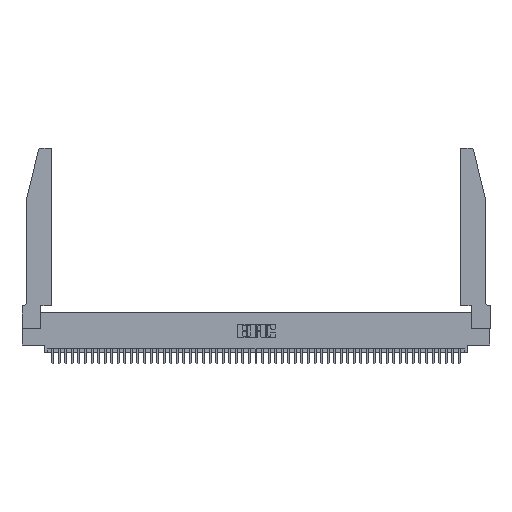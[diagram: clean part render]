
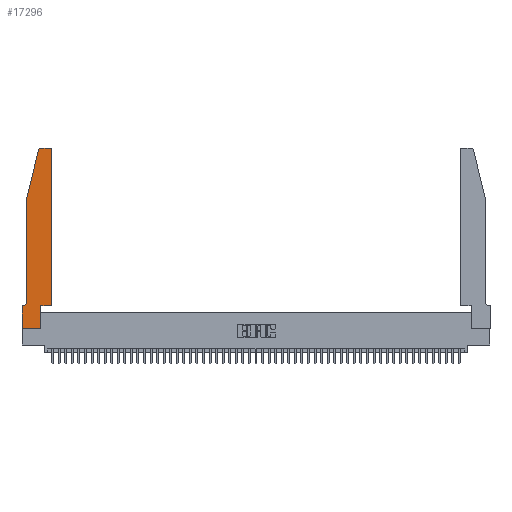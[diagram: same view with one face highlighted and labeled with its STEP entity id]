
A CAD part, top view. The second image highlights one B-rep face of the part: STEP entity #17296.
In plain terms, the highlighted planar face has unit normal (0, 0, 1).
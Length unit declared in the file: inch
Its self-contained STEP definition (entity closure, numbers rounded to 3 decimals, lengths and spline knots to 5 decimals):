
#713 = ORIENTED_EDGE ( 'NONE', *, *, #47006, .T. ) ;
#807 = EDGE_CURVE ( 'NONE', #51431, #30269, #21601, .T. ) ;
#2073 = ORIENTED_EDGE ( 'NONE', *, *, #3353, .T. ) ;
#3353 = EDGE_CURVE ( 'NONE', #23735, #6750, #13855, .T. ) ;
#3904 = VERTEX_POINT ( 'NONE', #6101 ) ;
#3996 = DIRECTION ( 'NONE',  ( 0., -1., 0. ) ) ;
#4215 = CARTESIAN_POINT ( 'NONE',  ( 0.0755, 2., 0.37 ) ) ;
#4515 = VERTEX_POINT ( 'NONE', #13367 ) ;
#4676 = CARTESIAN_POINT ( 'NONE',  ( 0.0755, 0.35, 0.37 ) ) ;
#4972 = CARTESIAN_POINT ( 'NONE',  ( 0.2865, 0.35, 0.37 ) ) ;
#5237 = PLANE ( 'NONE',  #23250 ) ;
#5437 = DIRECTION ( 'NONE',  ( 1., 0., 0. ) ) ;
#5572 = CARTESIAN_POINT ( 'NONE',  ( 0., 0., 0.37 ) ) ;
#5615 = DIRECTION ( 'NONE',  ( 0., 0., -1. ) ) ;
#5679 = DIRECTION ( 'NONE',  ( 1., 0., 0. ) ) ;
#5750 = ORIENTED_EDGE ( 'NONE', *, *, #49081, .T. ) ;
#6101 = CARTESIAN_POINT ( 'NONE',  ( 0.284, 2.75, 0.37 ) ) ;
#6127 = EDGE_CURVE ( 'NONE', #3904, #4515, #20749, .T. ) ;
#6750 = VERTEX_POINT ( 'NONE', #40614 ) ;
#6787 = CARTESIAN_POINT ( 'NONE',  ( 0.4505, 2.72, 0.37 ) ) ;
#8345 = EDGE_LOOP ( 'NONE', ( #8505, #27759, #46251, #5750, #2073, #32078, #30942, #51283, #11053, #10192, #48092, #713 ) ) ;
#8505 = ORIENTED_EDGE ( 'NONE', *, *, #30187, .T. ) ;
#8532 = CARTESIAN_POINT ( 'NONE',  ( 0.4205, 2.75, 0.37 ) ) ;
#9733 = EDGE_CURVE ( 'NONE', #40863, #49218, #51034, .T. ) ;
#9951 = CARTESIAN_POINT ( 'NONE',  ( 0.4205, 2.72, 0.37 ) ) ;
#10105 = LINE ( 'NONE', #41213, #39370 ) ;
#10192 = ORIENTED_EDGE ( 'NONE', *, *, #43537, .T. ) ;
#10645 = DIRECTION ( 'NONE',  ( 0., 0., 1. ) ) ;
#10842 = CARTESIAN_POINT ( 'NONE',  ( 0.4505, 0.35, 0.37 ) ) ;
#11053 = ORIENTED_EDGE ( 'NONE', *, *, #9733, .T. ) ;
#13268 = CARTESIAN_POINT ( 'NONE',  ( 0., 0.35, 0.37 ) ) ;
#13367 = CARTESIAN_POINT ( 'NONE',  ( 0.25487, 2.72718, 0.37 ) ) ;
#13855 = CIRCLE ( 'NONE', #32529, 0.07 ) ;
#14423 = EDGE_CURVE ( 'NONE', #4515, #18937, #43116, .T. ) ;
#14826 = DIRECTION ( 'NONE',  ( -1., 0., 0. ) ) ;
#16550 = DIRECTION ( 'NONE',  ( -1., 0., 0. ) ) ;
#16943 = VECTOR ( 'NONE', #47960, 39.37008 ) ;
#17296 = ADVANCED_FACE ( 'NONE', ( #25912 ), #5237, .T. ) ;
#17378 = AXIS2_PLACEMENT_3D ( 'NONE', #9951, #10645, #30489 ) ;
#18166 = VERTEX_POINT ( 'NONE', #31479 ) ;
#18937 = VERTEX_POINT ( 'NONE', #27567 ) ;
#20621 = CARTESIAN_POINT ( 'NONE',  ( 0.4505, 0.35, 0.37 ) ) ;
#20661 = DIRECTION ( 'NONE',  ( 0., 1., 0. ) ) ;
#20749 = CIRCLE ( 'NONE', #22957, 0.03 ) ;
#21378 = DIRECTION ( 'NONE',  ( 0., -1., 0. ) ) ;
#21601 = LINE ( 'NONE', #20621, #49634 ) ;
#22957 = AXIS2_PLACEMENT_3D ( 'NONE', #35944, #49182, #5437 ) ;
#23005 = VECTOR ( 'NONE', #20661, 39.37008 ) ;
#23250 = AXIS2_PLACEMENT_3D ( 'NONE', #13268, #41106, #33295 ) ;
#23680 = EDGE_CURVE ( 'NONE', #42241, #40863, #33078, .T. ) ;
#23735 = VERTEX_POINT ( 'NONE', #34259 ) ;
#25087 = DIRECTION ( 'NONE',  ( -1., 0., 0. ) ) ;
#25691 = DIRECTION ( 'NONE',  ( 1., 0., 0. ) ) ;
#25912 = FACE_OUTER_BOUND ( 'NONE', #8345, .T. ) ;
#27567 = CARTESIAN_POINT ( 'NONE',  ( 0.0755, 2., 0.37 ) ) ;
#27759 = ORIENTED_EDGE ( 'NONE', *, *, #6127, .T. ) ;
#27954 = LINE ( 'NONE', #30458, #47902 ) ;
#29962 = EDGE_CURVE ( 'NONE', #6750, #18166, #35785, .T. ) ;
#30187 = EDGE_CURVE ( 'NONE', #48262, #3904, #27954, .T. ) ;
#30269 = VERTEX_POINT ( 'NONE', #6787 ) ;
#30458 = CARTESIAN_POINT ( 'NONE',  ( 0.2605, 2.75, 0.37 ) ) ;
#30489 = DIRECTION ( 'NONE',  ( 1., 0., 0. ) ) ;
#30942 = ORIENTED_EDGE ( 'NONE', *, *, #48297, .T. ) ;
#31479 = CARTESIAN_POINT ( 'NONE',  ( 0., 0.35, 0.37 ) ) ;
#32078 = ORIENTED_EDGE ( 'NONE', *, *, #29962, .T. ) ;
#32127 = CIRCLE ( 'NONE', #17378, 0.03 ) ;
#32529 = AXIS2_PLACEMENT_3D ( 'NONE', #41301, #5615, #25087 ) ;
#33078 = LINE ( 'NONE', #49586, #43081 ) ;
#33254 = VECTOR ( 'NONE', #16550, 39.37008 ) ;
#33295 = DIRECTION ( 'NONE',  ( 1., 0., 0. ) ) ;
#33757 = CARTESIAN_POINT ( 'NONE',  ( 0.2865, 0., 0.37 ) ) ;
#34259 = CARTESIAN_POINT ( 'NONE',  ( 0.0755, 0.42, 0.37 ) ) ;
#35785 = LINE ( 'NONE', #4676, #33254 ) ;
#35944 = CARTESIAN_POINT ( 'NONE',  ( 0.284, 2.72, 0.37 ) ) ;
#36147 = LINE ( 'NONE', #45377, #38042 ) ;
#38042 = VECTOR ( 'NONE', #25691, 39.37008 ) ;
#39370 = VECTOR ( 'NONE', #21378, 39.37008 ) ;
#40025 = VECTOR ( 'NONE', #3996, 39.37008 ) ;
#40369 = CARTESIAN_POINT ( 'NONE',  ( 0., 0., 0.37 ) ) ;
#40614 = CARTESIAN_POINT ( 'NONE',  ( 0.0055, 0.35, 0.37 ) ) ;
#40863 = VERTEX_POINT ( 'NONE', #33757 ) ;
#41106 = DIRECTION ( 'NONE',  ( 0., 0., 1. ) ) ;
#41213 = CARTESIAN_POINT ( 'NONE',  ( 0.0755, 2., 0.37 ) ) ;
#41301 = CARTESIAN_POINT ( 'NONE',  ( 0.0055, 0.42, 0.37 ) ) ;
#41910 = CARTESIAN_POINT ( 'NONE',  ( 0.2865, 0.35, 0.37 ) ) ;
#42241 = VERTEX_POINT ( 'NONE', #5572 ) ;
#43081 = VECTOR ( 'NONE', #5679, 39.37008 ) ;
#43116 = LINE ( 'NONE', #4215, #16943 ) ;
#43537 = EDGE_CURVE ( 'NONE', #49218, #51431, #36147, .T. ) ;
#44150 = DIRECTION ( 'NONE',  ( 0., 1., 0. ) ) ;
#45377 = CARTESIAN_POINT ( 'NONE',  ( 0.4505, 0.35, 0.37 ) ) ;
#46251 = ORIENTED_EDGE ( 'NONE', *, *, #14423, .T. ) ;
#47006 = EDGE_CURVE ( 'NONE', #30269, #48262, #32127, .T. ) ;
#47902 = VECTOR ( 'NONE', #14826, 39.37008 ) ;
#47960 = DIRECTION ( 'NONE',  ( -0.239, -0.971, 0. ) ) ;
#48092 = ORIENTED_EDGE ( 'NONE', *, *, #807, .T. ) ;
#48262 = VERTEX_POINT ( 'NONE', #8532 ) ;
#48297 = EDGE_CURVE ( 'NONE', #18166, #42241, #50704, .T. ) ;
#49081 = EDGE_CURVE ( 'NONE', #18937, #23735, #10105, .T. ) ;
#49182 = DIRECTION ( 'NONE',  ( 0., 0., 1. ) ) ;
#49218 = VERTEX_POINT ( 'NONE', #41910 ) ;
#49586 = CARTESIAN_POINT ( 'NONE',  ( 0., 0., 0.37 ) ) ;
#49634 = VECTOR ( 'NONE', #44150, 39.37008 ) ;
#50704 = LINE ( 'NONE', #40369, #40025 ) ;
#51034 = LINE ( 'NONE', #4972, #23005 ) ;
#51283 = ORIENTED_EDGE ( 'NONE', *, *, #23680, .T. ) ;
#51431 = VERTEX_POINT ( 'NONE', #10842 ) ;
